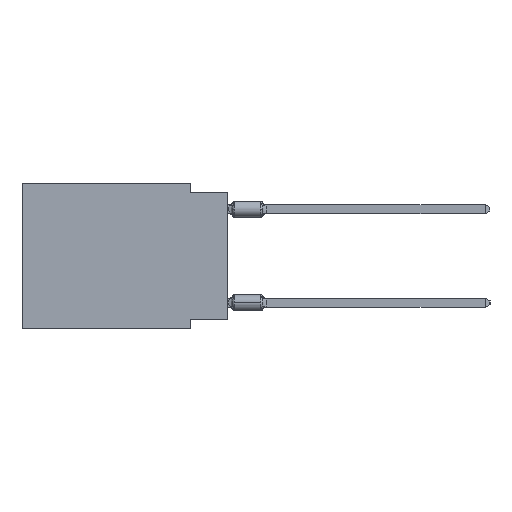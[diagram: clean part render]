
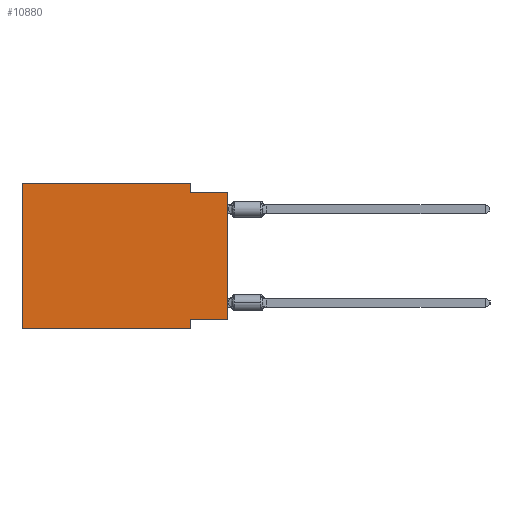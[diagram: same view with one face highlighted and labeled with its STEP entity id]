
A CAD part, left-side view. The second image highlights one B-rep face of the part: STEP entity #10880.
In plain terms, the highlighted planar face has unit normal (-1, 0, 0).
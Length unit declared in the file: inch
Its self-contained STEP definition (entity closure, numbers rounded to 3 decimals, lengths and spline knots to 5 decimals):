
#139 = CARTESIAN_POINT ( 'NONE',  ( 0., 0.55, 0. ) ) ;
#544 = CARTESIAN_POINT ( 'NONE',  ( 0., 0.55, 0. ) ) ;
#640 = ORIENTED_EDGE ( 'NONE', *, *, #36866, .F. ) ;
#692 = DIRECTION ( 'NONE',  ( 0., -1., 0. ) ) ;
#837 = DIRECTION ( 'NONE',  ( 0., -1., 0. ) ) ;
#2506 = CARTESIAN_POINT ( 'NONE',  ( 0., 0., -0.025 ) ) ;
#2659 = LINE ( 'NONE', #23890, #17842 ) ;
#3372 = DIRECTION ( 'NONE',  ( 0., 0., -1. ) ) ;
#3390 = VERTEX_POINT ( 'NONE', #7829 ) ;
#4684 = EDGE_CURVE ( 'NONE', #35072, #7678, #12912, .T. ) ;
#5946 = DIRECTION ( 'NONE',  ( 0., 0., -1. ) ) ;
#6742 = CARTESIAN_POINT ( 'NONE',  ( 0., 0.1, 0. ) ) ;
#6833 = DIRECTION ( 'NONE',  ( 0., 0., 1. ) ) ;
#7678 = VERTEX_POINT ( 'NONE', #21146 ) ;
#7829 = CARTESIAN_POINT ( 'NONE',  ( 0., 0.1, -0.365 ) ) ;
#8324 = VECTOR ( 'NONE', #18396, 39.37008 ) ;
#8593 = CARTESIAN_POINT ( 'NONE',  ( 0., 0.1, -0.025 ) ) ;
#8876 = ORIENTED_EDGE ( 'NONE', *, *, #24390, .F. ) ;
#9020 = VERTEX_POINT ( 'NONE', #8593 ) ;
#9778 = AXIS2_PLACEMENT_3D ( 'NONE', #139, #30810, #5946 ) ;
#10108 = EDGE_CURVE ( 'NONE', #25010, #17560, #21452, .T. ) ;
#10185 = EDGE_CURVE ( 'NONE', #14671, #31451, #10829, .T. ) ;
#10502 = CARTESIAN_POINT ( 'NONE',  ( 0., 0.55, -0.39 ) ) ;
#10634 = VECTOR ( 'NONE', #692, 39.37008 ) ;
#10829 = LINE ( 'NONE', #19644, #31503 ) ;
#10880 = ADVANCED_FACE ( 'NONE', ( #11949 ), #18556, .F. ) ;
#11949 = FACE_OUTER_BOUND ( 'NONE', #23995, .T. ) ;
#12438 = ORIENTED_EDGE ( 'NONE', *, *, #19446, .F. ) ;
#12912 = LINE ( 'NONE', #10502, #10634 ) ;
#12971 = CARTESIAN_POINT ( 'NONE',  ( 0., 0.55, -0.39 ) ) ;
#13191 = LINE ( 'NONE', #30844, #34527 ) ;
#13263 = VECTOR ( 'NONE', #15134, 39.37008 ) ;
#14671 = VERTEX_POINT ( 'NONE', #544 ) ;
#15134 = DIRECTION ( 'NONE',  ( 0., 0., 1. ) ) ;
#15746 = ORIENTED_EDGE ( 'NONE', *, *, #10108, .T. ) ;
#15972 = ORIENTED_EDGE ( 'NONE', *, *, #32891, .F. ) ;
#16247 = ORIENTED_EDGE ( 'NONE', *, *, #4684, .T. ) ;
#17560 = VERTEX_POINT ( 'NONE', #31934 ) ;
#17842 = VECTOR ( 'NONE', #38943, 39.37008 ) ;
#18396 = DIRECTION ( 'NONE',  ( 0., 1., 0. ) ) ;
#18556 = PLANE ( 'NONE',  #9778 ) ;
#19446 = EDGE_CURVE ( 'NONE', #9020, #17560, #35991, .T. ) ;
#19644 = CARTESIAN_POINT ( 'NONE',  ( 0., 0.55, 0. ) ) ;
#21146 = CARTESIAN_POINT ( 'NONE',  ( 0., 0.1, -0.39 ) ) ;
#21392 = CARTESIAN_POINT ( 'NONE',  ( 0., 0., -0.365 ) ) ;
#21452 = LINE ( 'NONE', #27698, #30213 ) ;
#23890 = CARTESIAN_POINT ( 'NONE',  ( 0., 0.1, -0.39 ) ) ;
#23995 = EDGE_LOOP ( 'NONE', ( #15746, #12438, #8876, #34066, #15972, #16247, #640, #24569 ) ) ;
#24197 = LINE ( 'NONE', #21392, #8324 ) ;
#24390 = EDGE_CURVE ( 'NONE', #31451, #9020, #13191, .T. ) ;
#24569 = ORIENTED_EDGE ( 'NONE', *, *, #25411, .F. ) ;
#25010 = VERTEX_POINT ( 'NONE', #36105 ) ;
#25148 = LINE ( 'NONE', #36573, #13263 ) ;
#25411 = EDGE_CURVE ( 'NONE', #25010, #3390, #24197, .T. ) ;
#27698 = CARTESIAN_POINT ( 'NONE',  ( 0., 0., 0. ) ) ;
#30213 = VECTOR ( 'NONE', #6833, 39.37008 ) ;
#30810 = DIRECTION ( 'NONE',  ( 1., 0., 0. ) ) ;
#30844 = CARTESIAN_POINT ( 'NONE',  ( 0., 0.1, 0. ) ) ;
#31451 = VERTEX_POINT ( 'NONE', #6742 ) ;
#31503 = VECTOR ( 'NONE', #837, 39.37008 ) ;
#31788 = VECTOR ( 'NONE', #33169, 39.37008 ) ;
#31934 = CARTESIAN_POINT ( 'NONE',  ( 0., 0., -0.025 ) ) ;
#32891 = EDGE_CURVE ( 'NONE', #35072, #14671, #25148, .T. ) ;
#33169 = DIRECTION ( 'NONE',  ( 0., -1., 0. ) ) ;
#34066 = ORIENTED_EDGE ( 'NONE', *, *, #10185, .F. ) ;
#34527 = VECTOR ( 'NONE', #3372, 39.37008 ) ;
#35072 = VERTEX_POINT ( 'NONE', #12971 ) ;
#35991 = LINE ( 'NONE', #2506, #31788 ) ;
#36105 = CARTESIAN_POINT ( 'NONE',  ( 0., 0., -0.365 ) ) ;
#36573 = CARTESIAN_POINT ( 'NONE',  ( 0., 0.55, 0. ) ) ;
#36866 = EDGE_CURVE ( 'NONE', #3390, #7678, #2659, .T. ) ;
#38943 = DIRECTION ( 'NONE',  ( 0., 0., -1. ) ) ;
